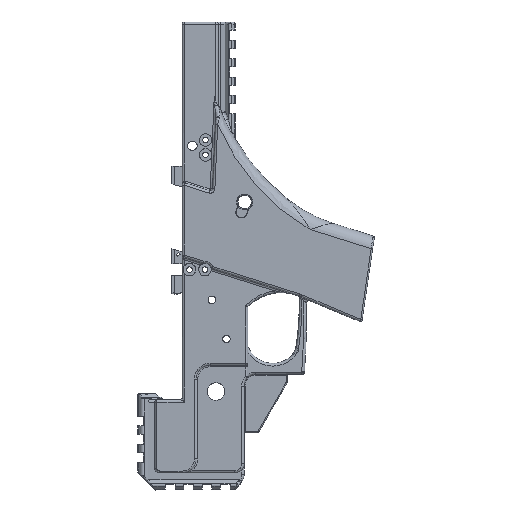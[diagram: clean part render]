
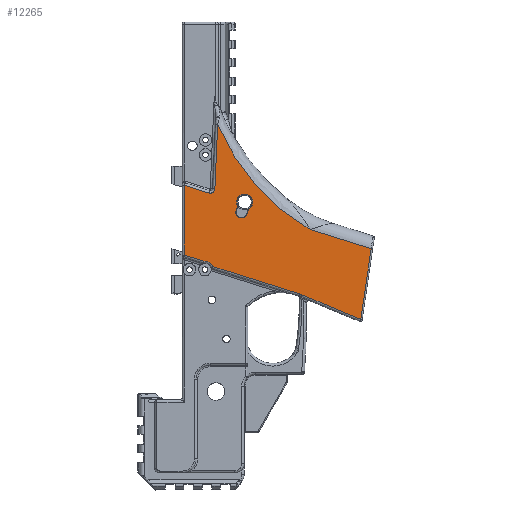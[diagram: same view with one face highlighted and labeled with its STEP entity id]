
A CAD part, left-side view. The second image highlights one B-rep face of the part: STEP entity #12265.
In plain terms, the highlighted planar face has unit normal (-1, 0, 0).
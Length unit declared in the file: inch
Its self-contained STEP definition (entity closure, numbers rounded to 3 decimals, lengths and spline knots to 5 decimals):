
#31=FACE_BOUND('',#3623,.T.);
#270=PLANE('',#13347);
#820=LINE('',#21297,#1703);
#841=LINE('',#21516,#1724);
#843=LINE('',#21537,#1726);
#845=LINE('',#21543,#1728);
#846=LINE('',#21545,#1729);
#847=LINE('',#21547,#1730);
#848=LINE('',#21551,#1731);
#849=LINE('',#21554,#1732);
#850=LINE('',#21558,#1733);
#851=LINE('',#21562,#1734);
#1703=VECTOR('',#15712,0.3937);
#1724=VECTOR('',#15763,0.3937);
#1726=VECTOR('',#15769,0.3937);
#1728=VECTOR('',#15775,0.3937);
#1729=VECTOR('',#15776,0.3937);
#1730=VECTOR('',#15777,0.3937);
#1731=VECTOR('',#15780,0.3937);
#1732=VECTOR('',#15783,0.3937);
#1733=VECTOR('',#15786,0.3937);
#1734=VECTOR('',#15789,0.3937);
#2873=FACE_OUTER_BOUND('',#3622,.T.);
#3622=EDGE_LOOP('',(#9636,#9637,#9638,#9639,#9640,#9641,#9642,#9643,#9644,
#9645,#9646,#9647));
#3623=EDGE_LOOP('',(#9648,#9649,#9650,#9651));
#4544=CIRCLE('',#13126,4.82183);
#4654=CIRCLE('',#13348,0.1845);
#4655=CIRCLE('',#13349,0.55);
#4656=CIRCLE('',#13350,0.1);
#4657=CIRCLE('',#13351,0.124);
#4658=CIRCLE('',#13352,0.1725);
#5370=VERTEX_POINT('',#20007);
#5371=VERTEX_POINT('',#20013);
#5567=VERTEX_POINT('',#21287);
#5569=VERTEX_POINT('',#21293);
#5603=VERTEX_POINT('',#21515);
#5605=VERTEX_POINT('',#21541);
#5606=VERTEX_POINT('',#21542);
#5607=VERTEX_POINT('',#21544);
#5608=VERTEX_POINT('',#21546);
#5609=VERTEX_POINT('',#21548);
#5610=VERTEX_POINT('',#21550);
#5611=VERTEX_POINT('',#21553);
#5612=VERTEX_POINT('',#21556);
#5613=VERTEX_POINT('',#21557);
#5614=VERTEX_POINT('',#21559);
#5615=VERTEX_POINT('',#21561);
#6724=EDGE_CURVE('',#5371,#5370,#4544,.T.);
#7025=EDGE_CURVE('',#5567,#5569,#820,.T.);
#7064=EDGE_CURVE('',#5569,#5603,#841,.T.);
#7068=EDGE_CURVE('',#5371,#5567,#843,.T.);
#7070=EDGE_CURVE('',#5605,#5606,#845,.T.);
#7071=EDGE_CURVE('',#5607,#5605,#846,.T.);
#7072=EDGE_CURVE('',#5608,#5607,#847,.T.);
#7073=EDGE_CURVE('',#5609,#5608,#4654,.T.);
#7074=EDGE_CURVE('',#5610,#5609,#848,.T.);
#7075=EDGE_CURVE('',#5603,#5610,#4655,.T.);
#7076=EDGE_CURVE('',#5611,#5370,#849,.T.);
#7077=EDGE_CURVE('',#5606,#5611,#4656,.T.);
#7078=EDGE_CURVE('',#5612,#5613,#850,.T.);
#7079=EDGE_CURVE('',#5614,#5612,#4657,.T.);
#7080=EDGE_CURVE('',#5615,#5614,#851,.T.);
#7081=EDGE_CURVE('',#5613,#5615,#4658,.T.);
#9636=ORIENTED_EDGE('',*,*,#7070,.F.);
#9637=ORIENTED_EDGE('',*,*,#7071,.F.);
#9638=ORIENTED_EDGE('',*,*,#7072,.F.);
#9639=ORIENTED_EDGE('',*,*,#7073,.F.);
#9640=ORIENTED_EDGE('',*,*,#7074,.F.);
#9641=ORIENTED_EDGE('',*,*,#7075,.F.);
#9642=ORIENTED_EDGE('',*,*,#7064,.F.);
#9643=ORIENTED_EDGE('',*,*,#7025,.F.);
#9644=ORIENTED_EDGE('',*,*,#7068,.F.);
#9645=ORIENTED_EDGE('',*,*,#6724,.T.);
#9646=ORIENTED_EDGE('',*,*,#7076,.F.);
#9647=ORIENTED_EDGE('',*,*,#7077,.F.);
#9648=ORIENTED_EDGE('',*,*,#7078,.F.);
#9649=ORIENTED_EDGE('',*,*,#7079,.F.);
#9650=ORIENTED_EDGE('',*,*,#7080,.F.);
#9651=ORIENTED_EDGE('',*,*,#7081,.F.);
#12265=ADVANCED_FACE('',(#2873,#31),#270,.T.);
#13126=AXIS2_PLACEMENT_3D('',#20014,#15163,#15164);
#13347=AXIS2_PLACEMENT_3D('',#21540,#15773,#15774);
#13348=AXIS2_PLACEMENT_3D('',#21549,#15778,#15779);
#13349=AXIS2_PLACEMENT_3D('',#21552,#15781,#15782);
#13350=AXIS2_PLACEMENT_3D('',#21555,#15784,#15785);
#13351=AXIS2_PLACEMENT_3D('',#21560,#15787,#15788);
#13352=AXIS2_PLACEMENT_3D('',#21563,#15790,#15791);
#15163=DIRECTION('center_axis',(1.,0.,0.));
#15164=DIRECTION('ref_axis',(0.,-0.858,0.513));
#15712=DIRECTION('',(0.,0.146,-0.989));
#15763=DIRECTION('',(0.,0.922,0.386));
#15769=DIRECTION('',(0.,-0.954,-0.301));
#15773=DIRECTION('center_axis',(-1.,0.,0.));
#15774=DIRECTION('ref_axis',(0.,0.301,-0.954));
#15775=DIRECTION('',(0.,-0.954,-0.301));
#15776=DIRECTION('',(0.,0.,1.));
#15777=DIRECTION('',(0.,0.954,0.301));
#15778=DIRECTION('center_axis',(-1.,0.,0.));
#15779=DIRECTION('ref_axis',(0.,-0.536,0.844));
#15780=DIRECTION('',(0.,0.954,0.301));
#15781=DIRECTION('center_axis',(-1.,0.,0.));
#15782=DIRECTION('ref_axis',(0.,-0.344,0.939));
#15783=DIRECTION('',(0.,-0.044,0.999));
#15784=DIRECTION('center_axis',(-1.,0.,0.));
#15785=DIRECTION('ref_axis',(0.,-0.574,-0.819));
#15786=DIRECTION('',(0.,-0.301,0.954));
#15787=DIRECTION('center_axis',(-1.,0.,0.));
#15788=DIRECTION('ref_axis',(0.,0.301,-0.954));
#15789=DIRECTION('',(0.,0.301,-0.954));
#15790=DIRECTION('center_axis',(-1.,0.,0.));
#15791=DIRECTION('ref_axis',(0.,-0.301,0.954));
#20007=CARTESIAN_POINT('',(-0.63,-0.54257,0.45432));
#20013=CARTESIAN_POINT('',(-0.63,-2.52341,-1.79711));
#20014=CARTESIAN_POINT('Origin',(-0.63,-4.97366,2.35575));
#21287=CARTESIAN_POINT('',(-0.63,-3.83543,-2.21079));
#21293=CARTESIAN_POINT('',(-0.63,-3.61188,-3.72465));
#21297=CARTESIAN_POINT('',(-0.63,-3.1983,-6.52542));
#21515=CARTESIAN_POINT('',(-0.63,-2.34601,-3.19423));
#21516=CARTESIAN_POINT('',(-0.63,-2.64354,-3.31889));
#21537=CARTESIAN_POINT('',(-0.63,-3.86992,-2.22167));
#21540=CARTESIAN_POINT('Origin',(-0.63,-3.86992,-2.22167));
#21541=CARTESIAN_POINT('',(-0.63,0.171,-0.84696));
#21542=CARTESIAN_POINT('',(-0.63,-0.35255,-1.01203));
#21543=CARTESIAN_POINT('',(-0.63,-1.83137,-1.4783));
#21544=CARTESIAN_POINT('',(-0.63,0.171,-2.34578));
#21545=CARTESIAN_POINT('',(-0.63,0.171,-0.68592));
#21546=CARTESIAN_POINT('',(-0.63,-0.23911,-2.47509));
#21547=CARTESIAN_POINT('',(-0.63,-1.92231,-3.0058));
#21548=CARTESIAN_POINT('',(-0.63,-0.44101,-2.59117));
#21549=CARTESIAN_POINT('Origin',(-0.63,-0.26873,
-2.6572));
#21550=CARTESIAN_POINT('',(-0.63,-2.29885,-3.17695));
#21551=CARTESIAN_POINT('',(-0.63,-3.45389,-3.54113));
#21552=CARTESIAN_POINT('Origin',(-0.63,-2.13346,-3.70149));
#21553=CARTESIAN_POINT('',(-0.63,-0.48252,-0.92102));
#21554=CARTESIAN_POINT('',(-0.63,-0.4624,-1.38187));
#21555=CARTESIAN_POINT('Origin',(-0.63,-0.38262,
-0.91666));
#21556=CARTESIAN_POINT('',(-0.63,-1.17219,-1.46199));
#21557=CARTESIAN_POINT('',(-0.63,-1.20439,-1.35986));
#21558=CARTESIAN_POINT('',(-0.63,-1.21936,-1.31239));
#21559=CARTESIAN_POINT('',(-0.63,-0.93567,-1.38741));
#21560=CARTESIAN_POINT('Origin',(-0.63,-1.05393,-1.4247));
#21561=CARTESIAN_POINT('',(-0.63,-0.96787,-1.28529));
#21562=CARTESIAN_POINT('',(-0.63,-0.9487,-1.34607));
#21563=CARTESIAN_POINT('Origin',(-0.63,-1.12219,-1.20821));
